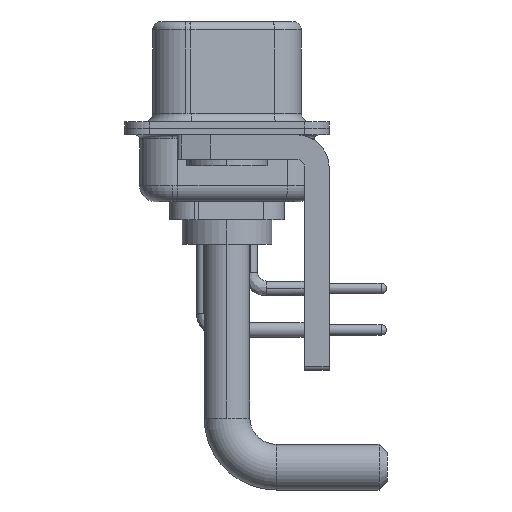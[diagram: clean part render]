
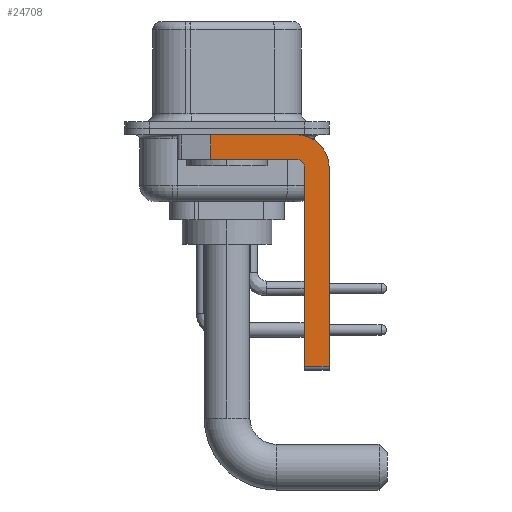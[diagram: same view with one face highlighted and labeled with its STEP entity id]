
A CAD part, left-side view. The second image highlights one B-rep face of the part: STEP entity #24708.
In plain terms, the highlighted planar face has unit normal (-1, 0, 0).
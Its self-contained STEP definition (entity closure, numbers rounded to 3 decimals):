
#93 = VECTOR ( 'NONE', #8300, 1000. ) ;
#380 = CARTESIAN_POINT ( 'NONE',  ( -2.9, -4.25, -14.55 ) ) ;
#758 = CARTESIAN_POINT ( 'NONE',  ( -2.9, -4.25, -2.4 ) ) ;
#823 = AXIS2_PLACEMENT_3D ( 'NONE', #5982, #9805, #13887 ) ;
#885 = EDGE_CURVE ( 'NONE', #7115, #14092, #17427, .T. ) ;
#1206 = DIRECTION ( 'NONE',  ( 0., 0., -1. ) ) ;
#1342 = CARTESIAN_POINT ( 'NONE',  ( -2.9, -4.75, -2.4 ) ) ;
#1612 = CARTESIAN_POINT ( 'NONE',  ( -2.9, 0.978, -1.9 ) ) ;
#2548 = VERTEX_POINT ( 'NONE', #1342 ) ;
#3200 = CARTESIAN_POINT ( 'NONE',  ( -2.9, -4.75, -14.55 ) ) ;
#3435 = CARTESIAN_POINT ( 'NONE',  ( -2.9, 3., -0.4 ) ) ;
#3578 = CARTESIAN_POINT ( 'NONE',  ( -2.9, -4.25, -1.9 ) ) ;
#4461 = VECTOR ( 'NONE', #21513, 1000. ) ;
#4590 = ORIENTED_EDGE ( 'NONE', *, *, #12022, .F. ) ;
#4790 = ORIENTED_EDGE ( 'NONE', *, *, #20304, .F. ) ;
#5076 = VERTEX_POINT ( 'NONE', #21930 ) ;
#5982 = CARTESIAN_POINT ( 'NONE',  ( -2.9, -4.25, -2.4 ) ) ;
#6058 = VECTOR ( 'NONE', #23082, 1000. ) ;
#6112 = CARTESIAN_POINT ( 'NONE',  ( -2.9, -6.25, -2.4 ) ) ;
#7115 = VERTEX_POINT ( 'NONE', #23413 ) ;
#7388 = LINE ( 'NONE', #3435, #6058 ) ;
#8036 = LINE ( 'NONE', #380, #93 ) ;
#8139 = FACE_OUTER_BOUND ( 'NONE', #13586, .T. ) ;
#8300 = DIRECTION ( 'NONE',  ( 0., -1., 0. ) ) ;
#8347 = VECTOR ( 'NONE', #13644, 1000. ) ;
#8600 = EDGE_CURVE ( 'NONE', #22882, #2548, #9885, .T. ) ;
#9805 = DIRECTION ( 'NONE',  ( 1., 0., 0. ) ) ;
#9885 = LINE ( 'NONE', #13841, #11489 ) ;
#10186 = ORIENTED_EDGE ( 'NONE', *, *, #885, .T. ) ;
#10884 = ORIENTED_EDGE ( 'NONE', *, *, #8600, .F. ) ;
#11071 = CARTESIAN_POINT ( 'NONE',  ( -2.9, -4.25, -1.9 ) ) ;
#11414 = CARTESIAN_POINT ( 'NONE',  ( -2.9, -6.25, -2.4 ) ) ;
#11489 = VECTOR ( 'NONE', #23160, 1000. ) ;
#11869 = LINE ( 'NONE', #3578, #14216 ) ;
#12022 = EDGE_CURVE ( 'NONE', #2548, #20617, #18655, .T. ) ;
#12267 = EDGE_CURVE ( 'NONE', #7115, #5076, #7388, .T. ) ;
#13586 = EDGE_LOOP ( 'NONE', ( #25007, #10186, #15029, #4590, #10884, #16205, #4790, #23240 ) ) ;
#13644 = DIRECTION ( 'NONE',  ( 0., 0., -1. ) ) ;
#13841 = CARTESIAN_POINT ( 'NONE',  ( -2.9, -4.75, -14.8 ) ) ;
#13887 = DIRECTION ( 'NONE',  ( 0., 0., -1. ) ) ;
#14092 = VERTEX_POINT ( 'NONE', #15386 ) ;
#14216 = VECTOR ( 'NONE', #19155, 1000. ) ;
#14668 = DIRECTION ( 'NONE',  ( 0., 0., 1. ) ) ;
#14804 = DIRECTION ( 'NONE',  ( -1., 0., 0. ) ) ;
#15029 = ORIENTED_EDGE ( 'NONE', *, *, #21702, .F. ) ;
#15386 = CARTESIAN_POINT ( 'NONE',  ( -2.9, 0.978, -1.9 ) ) ;
#15423 = AXIS2_PLACEMENT_3D ( 'NONE', #19078, #18694, #1206 ) ;
#15553 = PLANE ( 'NONE',  #823 ) ;
#16072 = LINE ( 'NONE', #6112, #8347 ) ;
#16205 = ORIENTED_EDGE ( 'NONE', *, *, #16439, .T. ) ;
#16439 = EDGE_CURVE ( 'NONE', #22882, #23049, #8036, .T. ) ;
#17427 = LINE ( 'NONE', #1612, #4461 ) ;
#18655 = CIRCLE ( 'NONE', #21527, 0.5 ) ;
#18694 = DIRECTION ( 'NONE',  ( 1., 0., 0. ) ) ;
#19078 = CARTESIAN_POINT ( 'NONE',  ( -2.9, -4.25, -2.4 ) ) ;
#19155 = DIRECTION ( 'NONE',  ( 0., 1., 0. ) ) ;
#19533 = CARTESIAN_POINT ( 'NONE',  ( -2.9, -6.25, -14.55 ) ) ;
#20304 = EDGE_CURVE ( 'NONE', #24282, #23049, #16072, .T. ) ;
#20617 = VERTEX_POINT ( 'NONE', #11071 ) ;
#21203 = EDGE_CURVE ( 'NONE', #5076, #24282, #24812, .T. ) ;
#21513 = DIRECTION ( 'NONE',  ( 0., 0., -1. ) ) ;
#21527 = AXIS2_PLACEMENT_3D ( 'NONE', #758, #14804, #14668 ) ;
#21702 = EDGE_CURVE ( 'NONE', #20617, #14092, #11869, .T. ) ;
#21930 = CARTESIAN_POINT ( 'NONE',  ( -2.9, -4.25, -0.4 ) ) ;
#22882 = VERTEX_POINT ( 'NONE', #3200 ) ;
#23049 = VERTEX_POINT ( 'NONE', #19533 ) ;
#23082 = DIRECTION ( 'NONE',  ( 0., -1., 0. ) ) ;
#23160 = DIRECTION ( 'NONE',  ( 0., 0., 1. ) ) ;
#23240 = ORIENTED_EDGE ( 'NONE', *, *, #21203, .F. ) ;
#23413 = CARTESIAN_POINT ( 'NONE',  ( -2.9, 0.978, -0.4 ) ) ;
#24282 = VERTEX_POINT ( 'NONE', #11414 ) ;
#24708 = ADVANCED_FACE ( 'NONE', ( #8139 ), #15553, .F. ) ;
#24812 = CIRCLE ( 'NONE', #15423, 2. ) ;
#25007 = ORIENTED_EDGE ( 'NONE', *, *, #12267, .F. ) ;
